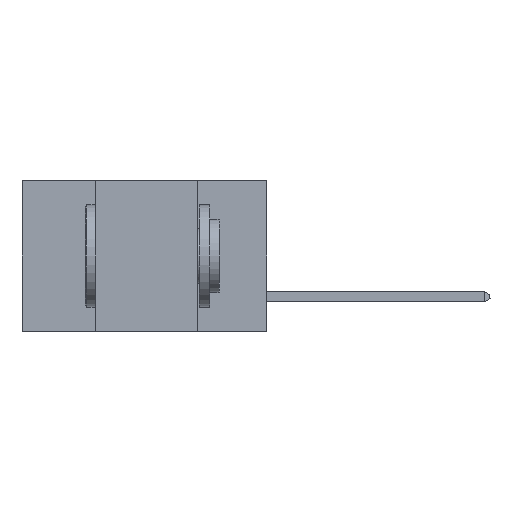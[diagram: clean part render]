
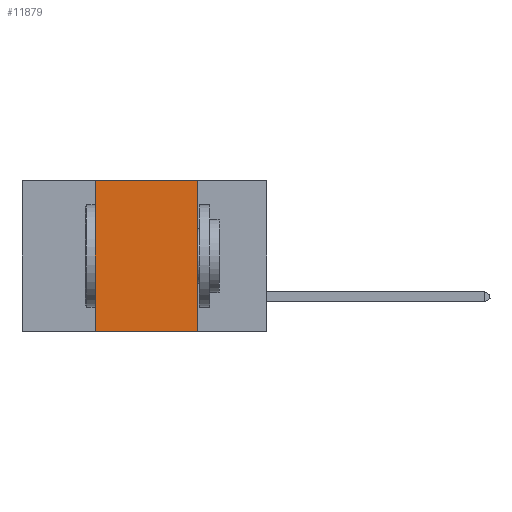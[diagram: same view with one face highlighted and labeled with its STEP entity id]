
A CAD part, left-side view. The second image highlights one B-rep face of the part: STEP entity #11879.
In plain terms, the highlighted planar face has unit normal (-1, 0, 0).
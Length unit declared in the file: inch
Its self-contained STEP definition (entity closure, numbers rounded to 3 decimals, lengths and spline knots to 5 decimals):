
#412 = EDGE_LOOP ( 'NONE', ( #1570, #1534, #11196, #14945 ) ) ;
#1534 = ORIENTED_EDGE ( 'NONE', *, *, #6856, .F. ) ;
#1570 = ORIENTED_EDGE ( 'NONE', *, *, #4129, .F. ) ;
#1762 = LINE ( 'NONE', #11615, #10790 ) ;
#2109 = DIRECTION ( 'NONE',  ( 0., -1., 0. ) ) ;
#3265 = EDGE_CURVE ( 'NONE', #7983, #11498, #1762, .T. ) ;
#3530 = LINE ( 'NONE', #4700, #16734 ) ;
#3574 = CARTESIAN_POINT ( 'NONE',  ( 0., 0.6, 0. ) ) ;
#4129 = EDGE_CURVE ( 'NONE', #5661, #7768, #3530, .T. ) ;
#4231 = LINE ( 'NONE', #3574, #6544 ) ;
#4347 = PLANE ( 'NONE',  #18389 ) ;
#4700 = CARTESIAN_POINT ( 'NONE',  ( 0., 0.17, 0. ) ) ;
#4897 = DIRECTION ( 'NONE',  ( 0., 0., -1. ) ) ;
#5026 = VECTOR ( 'NONE', #2109, 39.37008 ) ;
#5661 = VERTEX_POINT ( 'NONE', #9118 ) ;
#5758 = DIRECTION ( 'NONE',  ( 1., 0., 0. ) ) ;
#6544 = VECTOR ( 'NONE', #12110, 39.37008 ) ;
#6856 = EDGE_CURVE ( 'NONE', #11498, #5661, #4231, .T. ) ;
#7298 = DIRECTION ( 'NONE',  ( 0., 0., -1. ) ) ;
#7369 = FACE_OUTER_BOUND ( 'NONE', #412, .T. ) ;
#7768 = VERTEX_POINT ( 'NONE', #12972 ) ;
#7983 = VERTEX_POINT ( 'NONE', #9037 ) ;
#9037 = CARTESIAN_POINT ( 'NONE',  ( 0., 0.42, -0.37 ) ) ;
#9118 = CARTESIAN_POINT ( 'NONE',  ( 0., 0.17, 0. ) ) ;
#10790 = VECTOR ( 'NONE', #12866, 39.37008 ) ;
#11196 = ORIENTED_EDGE ( 'NONE', *, *, #3265, .F. ) ;
#11438 = CARTESIAN_POINT ( 'NONE',  ( 0., 0.6, 0. ) ) ;
#11498 = VERTEX_POINT ( 'NONE', #16323 ) ;
#11615 = CARTESIAN_POINT ( 'NONE',  ( 0., 0.42, 0. ) ) ;
#11879 = ADVANCED_FACE ( 'NONE', ( #7369 ), #4347, .F. ) ;
#12110 = DIRECTION ( 'NONE',  ( 0., -1., 0. ) ) ;
#12866 = DIRECTION ( 'NONE',  ( 0., 0., 1. ) ) ;
#12972 = CARTESIAN_POINT ( 'NONE',  ( 0., 0.17, -0.37 ) ) ;
#14359 = EDGE_CURVE ( 'NONE', #7983, #7768, #18669, .T. ) ;
#14945 = ORIENTED_EDGE ( 'NONE', *, *, #14359, .T. ) ;
#16323 = CARTESIAN_POINT ( 'NONE',  ( 0., 0.42, 0. ) ) ;
#16734 = VECTOR ( 'NONE', #4897, 39.37008 ) ;
#18065 = CARTESIAN_POINT ( 'NONE',  ( 0., 0.6, -0.37 ) ) ;
#18389 = AXIS2_PLACEMENT_3D ( 'NONE', #11438, #5758, #7298 ) ;
#18669 = LINE ( 'NONE', #18065, #5026 ) ;
